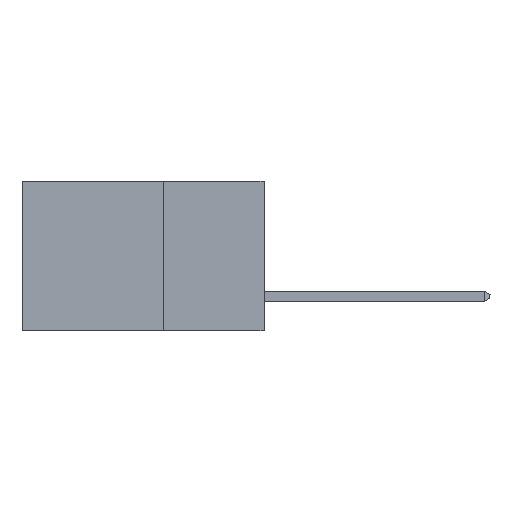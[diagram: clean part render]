
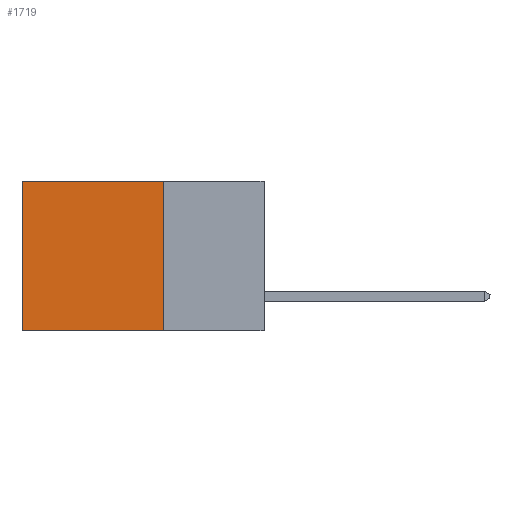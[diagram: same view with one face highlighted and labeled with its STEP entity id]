
A CAD part, left-side view. The second image highlights one B-rep face of the part: STEP entity #1719.
In plain terms, the highlighted planar face has unit normal (-1, 0, 0).
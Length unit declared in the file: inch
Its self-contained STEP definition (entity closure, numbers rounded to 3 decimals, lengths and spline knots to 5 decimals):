
#341 = DIRECTION ( 'NONE',  ( 0., 1., 0. ) ) ;
#1041 = VECTOR ( 'NONE', #1783, 39.37008 ) ;
#1249 = DIRECTION ( 'NONE',  ( 1., 0., 0. ) ) ;
#1405 = DIRECTION ( 'NONE',  ( 0., 0., -1. ) ) ;
#1719 = ADVANCED_FACE ( 'NONE', ( #7409 ), #5221, .F. ) ;
#1783 = DIRECTION ( 'NONE',  ( 0., 0., -1. ) ) ;
#1784 = EDGE_CURVE ( 'NONE', #6328, #4628, #8537, .T. ) ;
#1804 = CARTESIAN_POINT ( 'NONE',  ( 0.2615, 0.25, 0. ) ) ;
#2099 = EDGE_LOOP ( 'NONE', ( #5267, #9062, #7911, #5164 ) ) ;
#2214 = CARTESIAN_POINT ( 'NONE',  ( 0.2615, 0.25, -0.37 ) ) ;
#2637 = VERTEX_POINT ( 'NONE', #6365 ) ;
#3414 = VECTOR ( 'NONE', #1405, 39.37008 ) ;
#3488 = CARTESIAN_POINT ( 'NONE',  ( 0.2615, 0.25, 0. ) ) ;
#3675 = VERTEX_POINT ( 'NONE', #4105 ) ;
#3708 = VECTOR ( 'NONE', #341, 39.37008 ) ;
#4105 = CARTESIAN_POINT ( 'NONE',  ( 0.2615, 0.6, -0.37 ) ) ;
#4181 = CARTESIAN_POINT ( 'NONE',  ( 0.2615, 0.25, -0.37 ) ) ;
#4308 = LINE ( 'NONE', #9701, #1041 ) ;
#4519 = DIRECTION ( 'NONE',  ( 0., 1., 0. ) ) ;
#4628 = VERTEX_POINT ( 'NONE', #4181 ) ;
#5019 = VECTOR ( 'NONE', #4519, 39.37008 ) ;
#5164 = ORIENTED_EDGE ( 'NONE', *, *, #7945, .T. ) ;
#5221 = PLANE ( 'NONE',  #6561 ) ;
#5267 = ORIENTED_EDGE ( 'NONE', *, *, #8377, .T. ) ;
#6328 = VERTEX_POINT ( 'NONE', #1804 ) ;
#6365 = CARTESIAN_POINT ( 'NONE',  ( 0.2615, 0.6, 0. ) ) ;
#6561 = AXIS2_PLACEMENT_3D ( 'NONE', #6626, #1249, #9790 ) ;
#6597 = LINE ( 'NONE', #3488, #3708 ) ;
#6626 = CARTESIAN_POINT ( 'NONE',  ( 0.2615, 0.25, -0.37 ) ) ;
#6932 = CARTESIAN_POINT ( 'NONE',  ( 0.2615, 0.25, -0.37 ) ) ;
#6962 = LINE ( 'NONE', #2214, #5019 ) ;
#7409 = FACE_OUTER_BOUND ( 'NONE', #2099, .T. ) ;
#7911 = ORIENTED_EDGE ( 'NONE', *, *, #1784, .F. ) ;
#7945 = EDGE_CURVE ( 'NONE', #6328, #2637, #6597, .T. ) ;
#8377 = EDGE_CURVE ( 'NONE', #2637, #3675, #4308, .T. ) ;
#8537 = LINE ( 'NONE', #6932, #3414 ) ;
#9062 = ORIENTED_EDGE ( 'NONE', *, *, #9185, .F. ) ;
#9185 = EDGE_CURVE ( 'NONE', #4628, #3675, #6962, .T. ) ;
#9701 = CARTESIAN_POINT ( 'NONE',  ( 0.2615, 0.6, -0.37 ) ) ;
#9790 = DIRECTION ( 'NONE',  ( 0., 0., -1. ) ) ;
